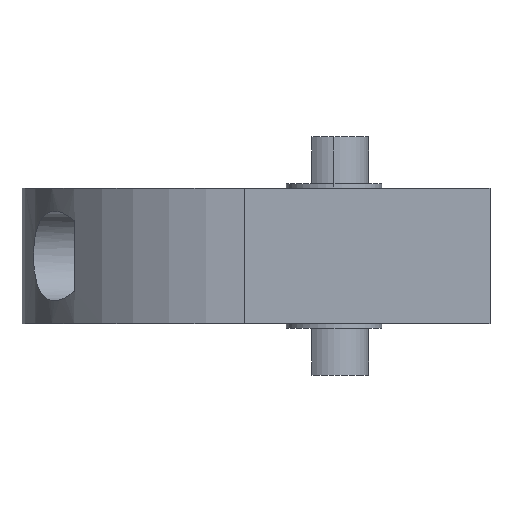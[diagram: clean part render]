
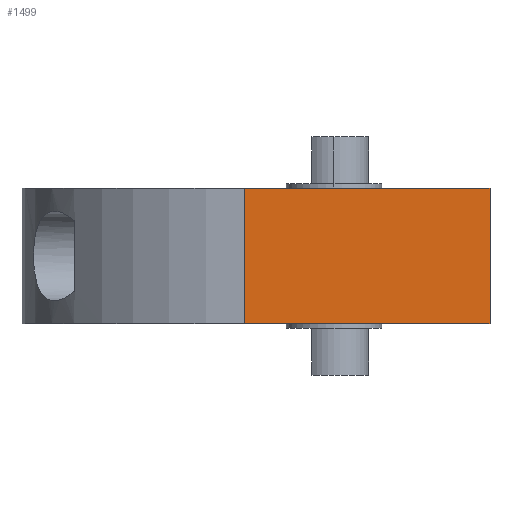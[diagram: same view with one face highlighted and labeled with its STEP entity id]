
A CAD part, left-side view. The second image highlights one B-rep face of the part: STEP entity #1499.
In plain terms, the highlighted planar face has unit normal (-1, 0, 0).
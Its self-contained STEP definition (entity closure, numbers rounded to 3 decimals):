
#57 = LINE ( 'NONE', #495, #672 ) ;
#95 = ORIENTED_EDGE ( 'NONE', *, *, #1538, .F. ) ;
#162 = VERTEX_POINT ( 'NONE', #1539 ) ;
#169 = VECTOR ( 'NONE', #646, 1000. ) ;
#326 = CARTESIAN_POINT ( 'NONE',  ( 0., 27.94, -15.494 ) ) ;
#407 = VERTEX_POINT ( 'NONE', #1350 ) ;
#441 = DIRECTION ( 'NONE',  ( 0., 0., -1. ) ) ;
#443 = CARTESIAN_POINT ( 'NONE',  ( 0., 27.94, 0. ) ) ;
#494 = DIRECTION ( 'NONE',  ( 0., 0., -1. ) ) ;
#495 = CARTESIAN_POINT ( 'NONE',  ( 0., 0., -15.494 ) ) ;
#501 = LINE ( 'NONE', #660, #169 ) ;
#552 = ORIENTED_EDGE ( 'NONE', *, *, #1668, .T. ) ;
#567 = VECTOR ( 'NONE', #441, 1000. ) ;
#646 = DIRECTION ( 'NONE',  ( 0., -1., 0. ) ) ;
#660 = CARTESIAN_POINT ( 'NONE',  ( 0., 0., 0. ) ) ;
#672 = VECTOR ( 'NONE', #494, 1000. ) ;
#691 = DIRECTION ( 'NONE',  ( 0., 1., 0. ) ) ;
#700 = CARTESIAN_POINT ( 'NONE',  ( 0., 25.4, -15.494 ) ) ;
#749 = DIRECTION ( 'NONE',  ( 0., 0., 1. ) ) ;
#750 = DIRECTION ( 'NONE',  ( -1., 0., 0. ) ) ;
#754 = CARTESIAN_POINT ( 'NONE',  ( 0., 0., 0. ) ) ;
#763 = PLANE ( 'NONE',  #786 ) ;
#786 = AXIS2_PLACEMENT_3D ( 'NONE', #754, #750, #749 ) ;
#940 = CARTESIAN_POINT ( 'NONE',  ( 0., 27.94, 0. ) ) ;
#984 = VECTOR ( 'NONE', #691, 1000. ) ;
#996 = LINE ( 'NONE', #443, #567 ) ;
#1008 = VERTEX_POINT ( 'NONE', #940 ) ;
#1181 = EDGE_LOOP ( 'NONE', ( #1504, #552, #95, #1327 ) ) ;
#1327 = ORIENTED_EDGE ( 'NONE', *, *, #1636, .F. ) ;
#1350 = CARTESIAN_POINT ( 'NONE',  ( 0., 0., -15.494 ) ) ;
#1393 = LINE ( 'NONE', #700, #984 ) ;
#1497 = FACE_OUTER_BOUND ( 'NONE', #1181, .T. ) ;
#1499 = ADVANCED_FACE ( 'NONE', ( #1497 ), #763, .T. ) ;
#1504 = ORIENTED_EDGE ( 'NONE', *, *, #1563, .F. ) ;
#1538 = EDGE_CURVE ( 'NONE', #407, #1771, #1393, .T. ) ;
#1539 = CARTESIAN_POINT ( 'NONE',  ( 0., 0., 0. ) ) ;
#1563 = EDGE_CURVE ( 'NONE', #1008, #162, #501, .T. ) ;
#1636 = EDGE_CURVE ( 'NONE', #162, #407, #57, .T. ) ;
#1668 = EDGE_CURVE ( 'NONE', #1008, #1771, #996, .T. ) ;
#1771 = VERTEX_POINT ( 'NONE', #326 ) ;
